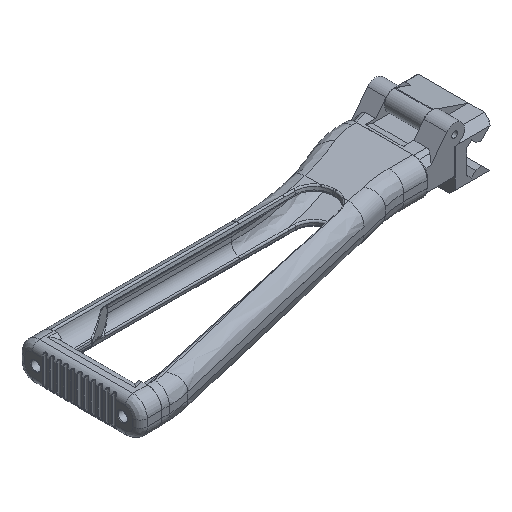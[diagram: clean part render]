
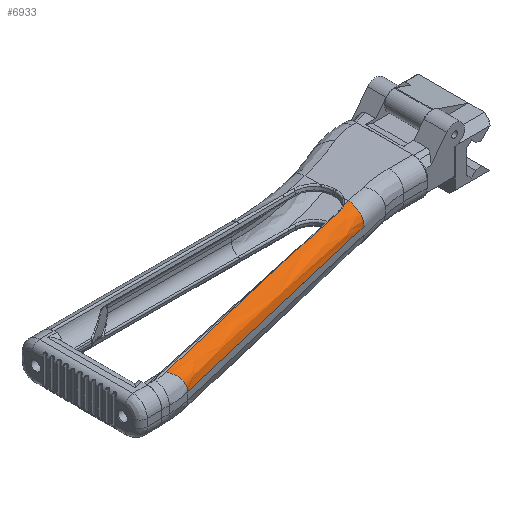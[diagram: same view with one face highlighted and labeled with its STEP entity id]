
A CAD part, isometric view. The second image highlights one B-rep face of the part: STEP entity #6933.
In plain terms, the highlighted free-form (B-spline) face has degree [2, 1] with [3, 2] control points.
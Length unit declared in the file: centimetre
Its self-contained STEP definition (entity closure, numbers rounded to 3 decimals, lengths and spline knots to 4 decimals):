
#84=(
BOUNDED_SURFACE()
B_SPLINE_SURFACE(2,1,((#14696,#14697),(#14698,#14699),(#14700,#14701)),
 .UNSPECIFIED.,.F.,.F.,.F.)
B_SPLINE_SURFACE_WITH_KNOTS((3,3),(2,2),(-1.5708,0.),
(0.,22.4136),.UNSPECIFIED.)
GEOMETRIC_REPRESENTATION_ITEM()
RATIONAL_B_SPLINE_SURFACE(((1.,1.),(0.707,0.707),
(1.,1.)))
REPRESENTATION_ITEM($)
SURFACE()
);
#331=B_SPLINE_CURVE_WITH_KNOTS($,3,(#14659,#14660,#14661,#14662),
 .UNSPECIFIED.,.F.,.F.,(4,4),(-0.5141,0.),.UNSPECIFIED.);
#333=B_SPLINE_CURVE_WITH_KNOTS($,3,(#14692,#14693,#14694,#14695),
 .UNSPECIFIED.,.F.,.F.,(4,4),(-5.6906,0.),.UNSPECIFIED.);
#334=B_SPLINE_CURVE_WITH_KNOTS($,3,(#14709,#14710,#14711,#14712,#14713,
#14714,#14715,#14716,#14717,#14718,#14719,#14720),.UNSPECIFIED.,.F.,.F.,
(4,2,2,2,2,4),(-1.6293,-1.4052,-1.1677,-0.7644,
-0.3743,0.),.UNSPECIFIED.);
#616=ELLIPSE($,#7507,1.0977,1.);
#895=FACE_OUTER_BOUND($,#1319,.T.);
#1319=EDGE_LOOP($,(#5693,#5694,#5695,#5696,#5697,#5698,#5699));
#2030=LINE($,#14703,#2501);
#2031=LINE($,#14707,#2502);
#2032=LINE($,#14721,#2503);
#2501=VECTOR($,#8836,10.3825);
#2502=VECTOR($,#8839,16.3705);
#2503=VECTOR($,#8840,0.3874);
#3135=VERTEX_POINT($,#14634);
#3136=VERTEX_POINT($,#14657);
#3138=VERTEX_POINT($,#14669);
#3139=VERTEX_POINT($,#14702);
#3140=VERTEX_POINT($,#14704);
#3141=VERTEX_POINT($,#14706);
#3142=VERTEX_POINT($,#14708);
#4044=EDGE_CURVE($,#3136,#3135,#331,.T.);
#4048=EDGE_CURVE($,#3138,#3136,#333,.T.);
#4049=EDGE_CURVE($,#3139,#3138,#2030,.T.);
#4050=EDGE_CURVE($,#3140,#3139,#616,.T.);
#4051=EDGE_CURVE($,#3141,#3140,#2031,.T.);
#4052=EDGE_CURVE($,#3142,#3141,#334,.T.);
#4053=EDGE_CURVE($,#3135,#3142,#2032,.T.);
#5693=ORIENTED_EDGE($,*,*,#4044,.F.);
#5694=ORIENTED_EDGE($,*,*,#4048,.F.);
#5695=ORIENTED_EDGE($,*,*,#4049,.F.);
#5696=ORIENTED_EDGE($,*,*,#4050,.F.);
#5697=ORIENTED_EDGE($,*,*,#4051,.F.);
#5698=ORIENTED_EDGE($,*,*,#4052,.F.);
#5699=ORIENTED_EDGE($,*,*,#4053,.F.);
#6933=ADVANCED_FACE($,(#895),#84,.F.);
#7507=AXIS2_PLACEMENT_3D($,#14705,#8837,#8838);
#8836=DIRECTION($,(0.973,0.232,0.));
#8837=DIRECTION('center_axis',(-0.851,-0.526,0.));
#8838=DIRECTION('ref_axis',(0.526,-0.851,0.));
#8839=DIRECTION($,(-0.973,-0.232,0.));
#8840=DIRECTION($,(0.973,0.232,0.));
#14634=CARTESIAN_POINT('',(-29.8402,-0.0354,41.6357));
#14657=CARTESIAN_POINT('',(-30.3086,-0.244,41.6316));
#14659=CARTESIAN_POINT('Ctrl Pts',(-30.3086,-0.244,
41.6316));
#14660=CARTESIAN_POINT('Ctrl Pts',(-30.1412,-0.207,
41.6314));
#14661=CARTESIAN_POINT('Ctrl Pts',(-29.9815,-0.1362,
41.6357));
#14662=CARTESIAN_POINT('Ctrl Pts',(-29.8402,-0.0354,
41.6357));
#14669=CARTESIAN_POINT('',(-35.8656,-1.4703,41.6357));
#14692=CARTESIAN_POINT('Ctrl Pts',(-35.8656,-1.4703,
41.6357));
#14693=CARTESIAN_POINT('Ctrl Pts',(-34.0133,-1.0617,
41.6357));
#14694=CARTESIAN_POINT('Ctrl Pts',(-32.1609,-0.6529,41.6343));
#14695=CARTESIAN_POINT('Ctrl Pts',(-30.3086,-0.244,
41.6316));
#14696=CARTESIAN_POINT('Ctrl Pts',(-27.7959,0.4514,
41.6357));
#14697=CARTESIAN_POINT('Ctrl Pts',(-49.5997,-4.741,
41.6357));
#14698=CARTESIAN_POINT('Ctrl Pts',(-27.5545,-0.5622,
41.6357));
#14699=CARTESIAN_POINT('Ctrl Pts',(-49.3583,-5.7546,
41.6357));
#14700=CARTESIAN_POINT('Ctrl Pts',(-27.5545,-0.5622,
40.6357));
#14701=CARTESIAN_POINT('Ctrl Pts',(-49.3583,-5.7546,40.6357));
#14702=CARTESIAN_POINT('',(-45.9657,-3.8756,41.6357));
#14703=CARTESIAN_POINT($,(-26.3884,0.7866,41.6357));
#14704=CARTESIAN_POINT('',(-45.3884,-4.8092,40.6357));
#14705=CARTESIAN_POINT('Origin',(-45.9657,-3.8756,40.6357));
#14706=CARTESIAN_POINT('',(-29.4633,-1.0167,40.6357));
#14707=CARTESIAN_POINT($,(-25.8111,-0.147,40.6357));
#14708=CARTESIAN_POINT('',(-29.4633,0.0544,41.6357));
#14709=CARTESIAN_POINT('Ctrl Pts',(-29.4633,0.0544,
41.6357));
#14710=CARTESIAN_POINT('Ctrl Pts',(-29.4633,-0.0205,
41.6357));
#14711=CARTESIAN_POINT('Ctrl Pts',(-29.4633,-0.0953,
41.6284));
#14712=CARTESIAN_POINT('Ctrl Pts',(-29.4633,-0.2465,
41.5983));
#14713=CARTESIAN_POINT('Ctrl Pts',(-29.4633,-0.3226,
41.5747));
#14714=CARTESIAN_POINT('Ctrl Pts',(-29.4633,-0.5191,
41.4898));
#14715=CARTESIAN_POINT('Ctrl Pts',(-29.4633,-0.6322,
41.4142));
#14716=CARTESIAN_POINT('Ctrl Pts',(-29.4633,-0.8197,
41.2272));
#14717=CARTESIAN_POINT('Ctrl Pts',(-29.4633,-0.8936,
41.1188));
#14718=CARTESIAN_POINT('Ctrl Pts',(-29.4633,-0.9917,
40.8836));
#14719=CARTESIAN_POINT('Ctrl Pts',(-29.4633,-1.0167,
40.7605));
#14720=CARTESIAN_POINT('Ctrl Pts',(-29.4633,-1.0167,
40.6357));
#14721=CARTESIAN_POINT($,(-26.3884,0.7866,41.6357));
